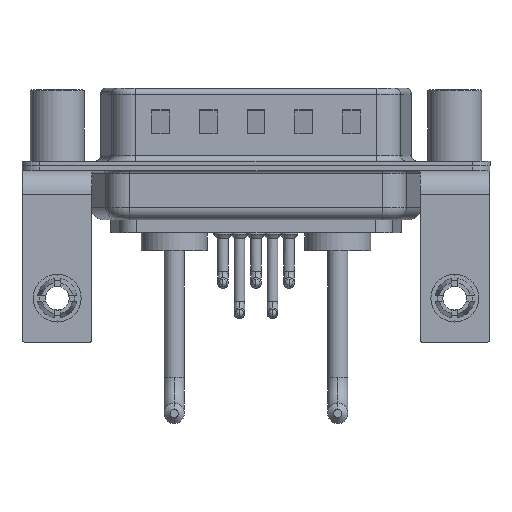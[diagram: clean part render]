
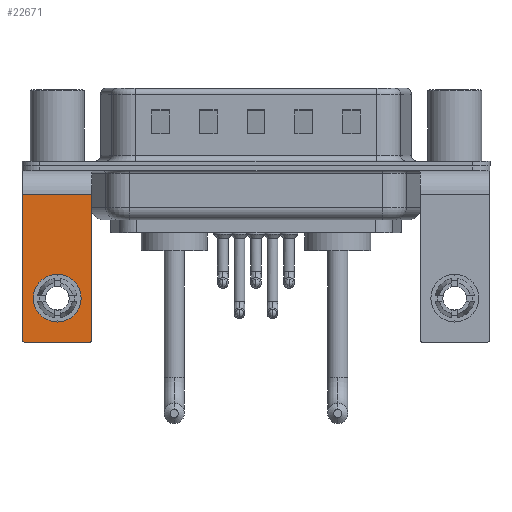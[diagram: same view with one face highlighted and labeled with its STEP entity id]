
A CAD part, front view. The second image highlights one B-rep face of the part: STEP entity #22671.
In plain terms, the highlighted planar face has unit normal (0, -1, 0).
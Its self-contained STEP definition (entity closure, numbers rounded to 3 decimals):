
#3 = VECTOR ( 'NONE', #11734, 1000. ) ;
#99 = CARTESIAN_POINT ( 'NONE',  ( 0., -6.25, -9.07 ) ) ;
#642 = EDGE_CURVE ( 'NONE', #13630, #10861, #8159, .T. ) ;
#758 = EDGE_CURVE ( 'NONE', #11976, #2393, #23745, .T. ) ;
#1498 = PLANE ( 'NONE',  #10176 ) ;
#1763 = DIRECTION ( 'NONE',  ( 0., 0., -1. ) ) ;
#2393 = VERTEX_POINT ( 'NONE', #9632 ) ;
#3745 = DIRECTION ( 'NONE',  ( 0., 0., 1. ) ) ;
#5296 = DIRECTION ( 'NONE',  ( 0., -1., 0. ) ) ;
#5691 = FACE_BOUND ( 'NONE', #16356, .T. ) ;
#6201 = VECTOR ( 'NONE', #1763, 1000. ) ;
#6318 = VERTEX_POINT ( 'NONE', #14256 ) ;
#7064 = DIRECTION ( 'NONE',  ( 0., 0., 1. ) ) ;
#7436 = FACE_OUTER_BOUND ( 'NONE', #14407, .T. ) ;
#7619 = ORIENTED_EDGE ( 'NONE', *, *, #19872, .F. ) ;
#7681 = CARTESIAN_POINT ( 'NONE',  ( -2.9, -6.25, -2.4 ) ) ;
#7725 = AXIS2_PLACEMENT_3D ( 'NONE', #18975, #13394, #17578 ) ;
#7953 = DIRECTION ( 'NONE',  ( 0., 1., 0. ) ) ;
#8132 = AXIS2_PLACEMENT_3D ( 'NONE', #19297, #13357, #21029 ) ;
#8159 = LINE ( 'NONE', #17937, #10300 ) ;
#8185 = CARTESIAN_POINT ( 'NONE',  ( -2.9, -6.25, -14.55 ) ) ;
#8399 = DIRECTION ( 'NONE',  ( -1., 0., 0. ) ) ;
#8715 = CARTESIAN_POINT ( 'NONE',  ( 2.65, -6.25, -14.8 ) ) ;
#9032 = CARTESIAN_POINT ( 'NONE',  ( 2.65, -6.25, -14.55 ) ) ;
#9632 = CARTESIAN_POINT ( 'NONE',  ( 2.9, -6.25, -14.55 ) ) ;
#9633 = CARTESIAN_POINT ( 'NONE',  ( 2.9, -6.25, -2.4 ) ) ;
#9820 = CARTESIAN_POINT ( 'NONE',  ( 0., -6.25, -11.07 ) ) ;
#9984 = VERTEX_POINT ( 'NONE', #23606 ) ;
#10176 = AXIS2_PLACEMENT_3D ( 'NONE', #24027, #20307, #7064 ) ;
#10265 = AXIS2_PLACEMENT_3D ( 'NONE', #9820, #7953, #3745 ) ;
#10300 = VECTOR ( 'NONE', #8399, 1000. ) ;
#10861 = VERTEX_POINT ( 'NONE', #7681 ) ;
#11108 = AXIS2_PLACEMENT_3D ( 'NONE', #9032, #5296, #16333 ) ;
#11182 = CARTESIAN_POINT ( 'NONE',  ( -2.9, -6.25, -2.4 ) ) ;
#11532 = CARTESIAN_POINT ( 'NONE',  ( 2.9, -6.25, -14.8 ) ) ;
#11734 = DIRECTION ( 'NONE',  ( 0., 0., -1. ) ) ;
#11976 = VERTEX_POINT ( 'NONE', #8715 ) ;
#12129 = EDGE_CURVE ( 'NONE', #10861, #22447, #17015, .T. ) ;
#13200 = CARTESIAN_POINT ( 'NONE',  ( 2.9, -6.25, -2.4 ) ) ;
#13357 = DIRECTION ( 'NONE',  ( 0., 1., 0. ) ) ;
#13387 = DIRECTION ( 'NONE',  ( -1., 0., 0. ) ) ;
#13394 = DIRECTION ( 'NONE',  ( 0., -1., 0. ) ) ;
#13630 = VERTEX_POINT ( 'NONE', #13200 ) ;
#14256 = CARTESIAN_POINT ( 'NONE',  ( 0., -6.25, -13.07 ) ) ;
#14407 = EDGE_LOOP ( 'NONE', ( #22931, #24208, #16173, #24342, #7619, #14668 ) ) ;
#14458 = CIRCLE ( 'NONE', #8132, 2. ) ;
#14668 = ORIENTED_EDGE ( 'NONE', *, *, #642, .T. ) ;
#15050 = VERTEX_POINT ( 'NONE', #99 ) ;
#15904 = EDGE_CURVE ( 'NONE', #15050, #6318, #17386, .T. ) ;
#16173 = ORIENTED_EDGE ( 'NONE', *, *, #19460, .F. ) ;
#16333 = DIRECTION ( 'NONE',  ( 0., 0., 1. ) ) ;
#16356 = EDGE_LOOP ( 'NONE', ( #17396, #20859 ) ) ;
#17015 = LINE ( 'NONE', #11182, #6201 ) ;
#17386 = CIRCLE ( 'NONE', #10265, 2. ) ;
#17396 = ORIENTED_EDGE ( 'NONE', *, *, #21262, .T. ) ;
#17578 = DIRECTION ( 'NONE',  ( 0., 0., 1. ) ) ;
#17937 = CARTESIAN_POINT ( 'NONE',  ( 2.9, -6.25, -2.4 ) ) ;
#18975 = CARTESIAN_POINT ( 'NONE',  ( -2.65, -6.25, -14.55 ) ) ;
#19159 = LINE ( 'NONE', #9633, #3 ) ;
#19297 = CARTESIAN_POINT ( 'NONE',  ( 0., -6.25, -11.07 ) ) ;
#19460 = EDGE_CURVE ( 'NONE', #11976, #9984, #23026, .T. ) ;
#19872 = EDGE_CURVE ( 'NONE', #13630, #2393, #19159, .T. ) ;
#20307 = DIRECTION ( 'NONE',  ( 0., 1., 0. ) ) ;
#20537 = VECTOR ( 'NONE', #13387, 1000. ) ;
#20859 = ORIENTED_EDGE ( 'NONE', *, *, #15904, .T. ) ;
#20866 = EDGE_CURVE ( 'NONE', #22447, #9984, #23534, .T. ) ;
#21029 = DIRECTION ( 'NONE',  ( 0., 0., 1. ) ) ;
#21262 = EDGE_CURVE ( 'NONE', #6318, #15050, #14458, .T. ) ;
#22447 = VERTEX_POINT ( 'NONE', #8185 ) ;
#22671 = ADVANCED_FACE ( 'NONE', ( #5691, #7436 ), #1498, .F. ) ;
#22931 = ORIENTED_EDGE ( 'NONE', *, *, #12129, .T. ) ;
#23026 = LINE ( 'NONE', #11532, #20537 ) ;
#23534 = CIRCLE ( 'NONE', #7725, 0.25 ) ;
#23606 = CARTESIAN_POINT ( 'NONE',  ( -2.65, -6.25, -14.8 ) ) ;
#23745 = CIRCLE ( 'NONE', #11108, 0.25 ) ;
#24027 = CARTESIAN_POINT ( 'NONE',  ( 2.9, -6.25, -2.4 ) ) ;
#24208 = ORIENTED_EDGE ( 'NONE', *, *, #20866, .T. ) ;
#24342 = ORIENTED_EDGE ( 'NONE', *, *, #758, .T. ) ;
